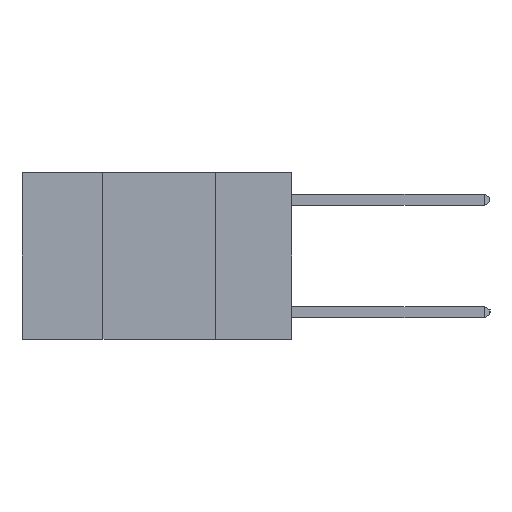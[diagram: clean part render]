
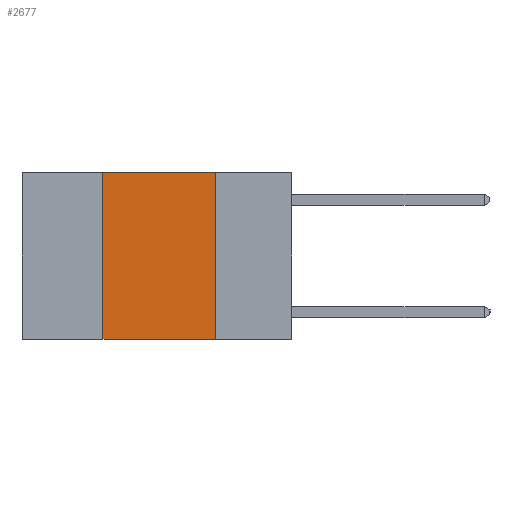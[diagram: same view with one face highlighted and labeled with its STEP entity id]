
A CAD part, left-side view. The second image highlights one B-rep face of the part: STEP entity #2677.
In plain terms, the highlighted planar face has unit normal (-1, 0, 0).
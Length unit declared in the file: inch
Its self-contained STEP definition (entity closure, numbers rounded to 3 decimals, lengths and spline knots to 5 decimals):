
#195 = EDGE_LOOP ( 'NONE', ( #1845, #9016, #2409, #8115 ) ) ;
#781 = LINE ( 'NONE', #1202, #1048 ) ;
#937 = DIRECTION ( 'NONE',  ( 0., -1., 0. ) ) ;
#1048 = VECTOR ( 'NONE', #937, 39.37008 ) ;
#1075 = EDGE_CURVE ( 'NONE', #8718, #3666, #9934, .T. ) ;
#1202 = CARTESIAN_POINT ( 'NONE',  ( 0., 0.6, -0.37 ) ) ;
#1710 = AXIS2_PLACEMENT_3D ( 'NONE', #8190, #8160, #8132 ) ;
#1845 = ORIENTED_EDGE ( 'NONE', *, *, #1075, .F. ) ;
#2249 = LINE ( 'NONE', #3631, #9120 ) ;
#2331 = CARTESIAN_POINT ( 'NONE',  ( 0., 0.17, 0. ) ) ;
#2409 = ORIENTED_EDGE ( 'NONE', *, *, #5080, .F. ) ;
#2677 = ADVANCED_FACE ( 'NONE', ( #6925 ), #8358, .F. ) ;
#2892 = CARTESIAN_POINT ( 'NONE',  ( 0., 0.17, 0. ) ) ;
#2898 = EDGE_CURVE ( 'NONE', #4901, #3666, #781, .T. ) ;
#3631 = CARTESIAN_POINT ( 'NONE',  ( 0., 0.6, 0. ) ) ;
#3666 = VERTEX_POINT ( 'NONE', #5659 ) ;
#4285 = CARTESIAN_POINT ( 'NONE',  ( 0., 0.42, 0. ) ) ;
#4901 = VERTEX_POINT ( 'NONE', #5721 ) ;
#5080 = EDGE_CURVE ( 'NONE', #4901, #6390, #6351, .T. ) ;
#5220 = CARTESIAN_POINT ( 'NONE',  ( 0., 0.42, 0. ) ) ;
#5659 = CARTESIAN_POINT ( 'NONE',  ( 0., 0.17, -0.37 ) ) ;
#5721 = CARTESIAN_POINT ( 'NONE',  ( 0., 0.42, -0.37 ) ) ;
#5807 = EDGE_CURVE ( 'NONE', #6390, #8718, #2249, .T. ) ;
#6115 = DIRECTION ( 'NONE',  ( 0., 0., 1. ) ) ;
#6351 = LINE ( 'NONE', #4285, #8647 ) ;
#6390 = VERTEX_POINT ( 'NONE', #5220 ) ;
#6925 = FACE_OUTER_BOUND ( 'NONE', #195, .T. ) ;
#7774 = VECTOR ( 'NONE', #7959, 39.37008 ) ;
#7959 = DIRECTION ( 'NONE',  ( 0., 0., -1. ) ) ;
#8115 = ORIENTED_EDGE ( 'NONE', *, *, #2898, .T. ) ;
#8132 = DIRECTION ( 'NONE',  ( 0., 0., -1. ) ) ;
#8160 = DIRECTION ( 'NONE',  ( 1., 0., 0. ) ) ;
#8190 = CARTESIAN_POINT ( 'NONE',  ( 0., 0.6, 0. ) ) ;
#8358 = PLANE ( 'NONE',  #1710 ) ;
#8647 = VECTOR ( 'NONE', #6115, 39.37008 ) ;
#8718 = VERTEX_POINT ( 'NONE', #2892 ) ;
#9016 = ORIENTED_EDGE ( 'NONE', *, *, #5807, .F. ) ;
#9120 = VECTOR ( 'NONE', #10504, 39.37008 ) ;
#9934 = LINE ( 'NONE', #2331, #7774 ) ;
#10504 = DIRECTION ( 'NONE',  ( 0., -1., 0. ) ) ;
